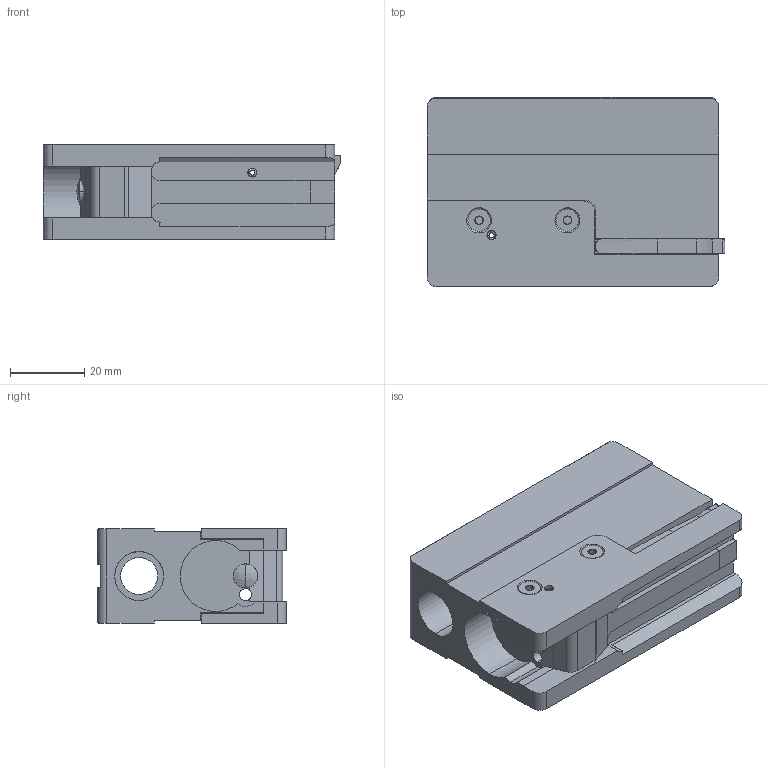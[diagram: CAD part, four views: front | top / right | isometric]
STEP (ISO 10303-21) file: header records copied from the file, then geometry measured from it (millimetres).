
FILE_DESCRIPTION (( 'STEP AP214' ), '1' );
FILE_NAME ('PPDW9 V2 Split Bolt.STEP', '2020-12-28T02:52:50', ( '' ), ( '' ), 'SwSTEP 2.0', 'SolidWorks 2020', '' );
FILE_SCHEMA (( 'AUTOMOTIVE_DESIGN' ));
Length unit declared in the file: inch
Products named in the file (10): PPDW9 V2 Split Bolt 2 piece; PPDW9 V2 Split Bolt bottom; Extractor spring 9657K256_9657K256; PPDW9 V2 Split Bolt upper; Beretta 92 scanned extractor; PPDW9 V2 Split Bolt; M3 x 6mm FHSHS 91294A126_BLACK_91294A126; 3-32 92383A859_TYPE 420 STAINLESS STEEL SLOTTED SPRING PIN_92383A859; P38 Firing Pin; Firing Pin Spring 9657K242_9657K242
Assembly tree (13 placements, depth 3):
  PPDW9 V2 Split Bolt
    PPDW9 V2 Split Bolt 2 piece
      PPDW9 V2 Split Bolt upper
      PPDW9 V2 Split Bolt bottom
    P38 Firing Pin
    Extractor spring 9657K256_9657K256
    Firing Pin Spring 9657K242_9657K242
    3-32 92383A859_TYPE 420 STAINLESS STEEL SLOTTED SPRING PIN_92383A859  x2
    Beretta 92 scanned extractor
    M3 x 6mm FHSHS 91294A126_BLACK_91294A126  x4
Bounding box: 79.99 x 50.8 x 25.4 mm (x, y, z)
Volume: 76424.8 mm3; surface area: 31705.1 mm2
Topology: 12 solids, 12 shells, 572 faces, 1518 edges, 964 vertices
Faces by surface type: cylinder 260, plane 177, cone 82, bspline 38, torus 9, sphere 6
Entity records: 22224 total; most frequent: CARTESIAN_POINT 12353, ORIENTED_EDGE 2036, DIRECTION 1844, EDGE_CURVE 1018, AXIS2_PLACEMENT_3D 667, VERTEX_POINT 654, VECTOR 510, LINE 510
